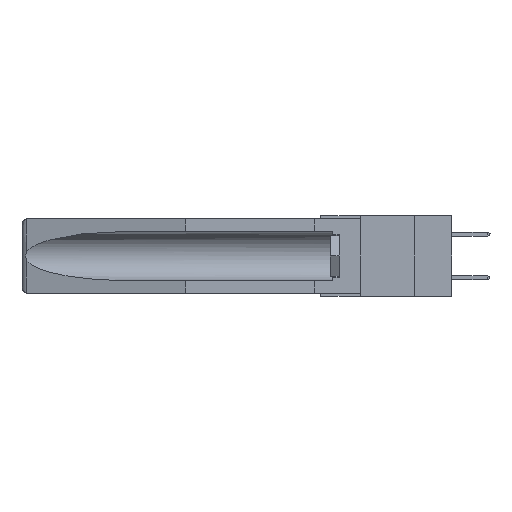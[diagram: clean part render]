
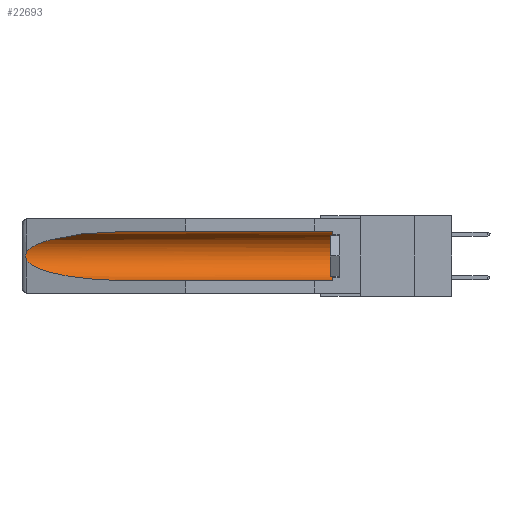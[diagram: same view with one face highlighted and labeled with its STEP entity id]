
A CAD part, left-side view. The second image highlights one B-rep face of the part: STEP entity #22693.
In plain terms, the highlighted cylindrical face has radius 2.857 mm (diameter 5.715 mm), a partial arc.
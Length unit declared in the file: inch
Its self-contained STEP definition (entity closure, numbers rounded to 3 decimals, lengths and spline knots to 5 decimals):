
#104 = DIRECTION ( 'NONE',  ( 0., 0., 1. ) ) ;
#618 = VERTEX_POINT ( 'NONE', #13169 ) ;
#2850 = AXIS2_PLACEMENT_3D ( 'NONE', #29302, #12072, #104 ) ;
#3590 = VERTEX_POINT ( 'NONE', #14461 ) ;
#4491 = EDGE_CURVE ( 'NONE', #618, #12847, #23734, .T. ) ;
#5005 = DIRECTION ( 'NONE',  ( 0., 1., 0. ) ) ;
#6200 = ORIENTED_EDGE ( 'NONE', *, *, #6439, .T. ) ;
#6439 = EDGE_CURVE ( 'NONE', #16627, #12847, #22636, .T. ) ;
#6480 = CARTESIAN_POINT ( 'NONE',  ( 0.21114, 1.30732, -0.059 ) ) ;
#6507 = CARTESIAN_POINT ( 'NONE',  ( 0.26537, 1.52718, -0.19328 ) ) ;
#8005 = LINE ( 'NONE', #29593, #15576 ) ;
#9038 = CARTESIAN_POINT ( 'NONE',  ( 0.155, -0.30754, -0.284 ) ) ;
#10639 = CARTESIAN_POINT ( 'NONE',  ( 0.155, 1.07973, -0.284 ) ) ;
#10770 = EDGE_LOOP ( 'NONE', ( #22137, #22487, #6200, #28741, #30874, #13702 ) ) ;
#10955 = CARTESIAN_POINT ( 'NONE',  ( 0.2673, 1.53269, -0.17917 ) ) ;
#11269 = CARTESIAN_POINT ( 'NONE',  ( 0.26655, 1.53094, -0.18657 ) ) ;
#11281 = VECTOR ( 'NONE', #30518, 39.37008 ) ;
#12072 = DIRECTION ( 'NONE',  ( 0., -1., 0. ) ) ;
#12361 = EDGE_CURVE ( 'NONE', #618, #3590, #28102, .T. ) ;
#12847 = VERTEX_POINT ( 'NONE', #10639 ) ;
#12888 = DIRECTION ( 'NONE',  ( 0., 1., 0. ) ) ;
#13169 = CARTESIAN_POINT ( 'NONE',  ( 0.155, 0.126, -0.284 ) ) ;
#13183 = CARTESIAN_POINT ( 'NONE',  ( 0.26597, 1.52961, -0.15275 ) ) ;
#13702 = ORIENTED_EDGE ( 'NONE', *, *, #24651, .T. ) ;
#14461 = CARTESIAN_POINT ( 'NONE',  ( 0.155, 0.126, -0.059 ) ) ;
#15488 = CARTESIAN_POINT ( 'NONE',  ( 0.26537, 1.52718, -0.19328 ) ) ;
#15576 = VECTOR ( 'NONE', #12888, 39.37008 ) ;
#15831 = CARTESIAN_POINT ( 'NONE',  ( 0.26537, 1.52718, -0.19328 ) ) ;
#16154 = CARTESIAN_POINT ( 'NONE',  ( 0.26597, 1.5296, -0.19026 ) ) ;
#16467 =( BOUNDED_CURVE ( )  B_SPLINE_CURVE ( 3, ( #31258, #6480, #23387, #16859 ),
 .UNSPECIFIED., .F., .T. ) 
 B_SPLINE_CURVE_WITH_KNOTS ( ( 4, 4 ),
 ( 4.71239, 6.08839 ),
 .UNSPECIFIED. ) 
 CURVE ( )  GEOMETRIC_REPRESENTATION_ITEM ( )  RATIONAL_B_SPLINE_CURVE ( ( 1., 0.848, 0.848, 1. ) ) 
 REPRESENTATION_ITEM ( '' )  );
#16627 = VERTEX_POINT ( 'NONE', #15488 ) ;
#16859 = CARTESIAN_POINT ( 'NONE',  ( 0.26537, 1.52718, -0.14972 ) ) ;
#17693 = EDGE_CURVE ( 'NONE', #24931, #26685, #16467, .T. ) ;
#17947 = CARTESIAN_POINT ( 'NONE',  ( 0.26537, 1.52718, -0.14972 ) ) ;
#19496 = EDGE_CURVE ( 'NONE', #26685, #16627, #21074, .T. ) ;
#19726 = CARTESIAN_POINT ( 'NONE',  ( 0.155, -0.30754, -0.1715 ) ) ;
#20788 = CARTESIAN_POINT ( 'NONE',  ( 0.2675, 1.53308, -0.16763 ) ) ;
#20820 = CARTESIAN_POINT ( 'NONE',  ( 0.26537, 1.52718, -0.14972 ) ) ;
#21074 = B_SPLINE_CURVE_WITH_KNOTS ( 'NONE', 3,
 ( #17947, #13183, #28186, #30318, #20788, #25516, #10955, #11269, #16154, #6507 ),
 .UNSPECIFIED., .F., .F.,
 ( 4, 2, 2, 2, 4 ),
 ( 0., 0.00029, 0.00058, 0.00087, 0.00117 ),
 .UNSPECIFIED. ) ;
#22137 = ORIENTED_EDGE ( 'NONE', *, *, #17693, .T. ) ;
#22348 = DIRECTION ( 'NONE',  ( 0., 0., 1. ) ) ;
#22487 = ORIENTED_EDGE ( 'NONE', *, *, #19496, .T. ) ;
#22636 =( BOUNDED_CURVE ( )  B_SPLINE_CURVE ( 3, ( #15831, #27751, #25714, #27970 ),
 .UNSPECIFIED., .F., .F. ) 
 B_SPLINE_CURVE_WITH_KNOTS ( ( 4, 4 ),
 ( 0.1948, 1.5708 ),
 .UNSPECIFIED. ) 
 CURVE ( )  GEOMETRIC_REPRESENTATION_ITEM ( )  RATIONAL_B_SPLINE_CURVE ( ( 1., 0.848, 0.848, 1. ) ) 
 REPRESENTATION_ITEM ( '' )  );
#22693 = ADVANCED_FACE ( 'NONE', ( #28158 ), #24349, .F. ) ;
#23387 = CARTESIAN_POINT ( 'NONE',  ( 0.25451, 1.48313, -0.09465 ) ) ;
#23734 = LINE ( 'NONE', #9038, #11281 ) ;
#24349 = CYLINDRICAL_SURFACE ( 'NONE', #30832, 0.1125 ) ;
#24651 = EDGE_CURVE ( 'NONE', #3590, #24931, #8005, .T. ) ;
#24931 = VERTEX_POINT ( 'NONE', #31096 ) ;
#25516 = CARTESIAN_POINT ( 'NONE',  ( 0.2675, 1.53308, -0.17534 ) ) ;
#25714 = CARTESIAN_POINT ( 'NONE',  ( 0.21114, 1.30732, -0.284 ) ) ;
#26685 = VERTEX_POINT ( 'NONE', #20820 ) ;
#27751 = CARTESIAN_POINT ( 'NONE',  ( 0.25451, 1.48313, -0.24835 ) ) ;
#27970 = CARTESIAN_POINT ( 'NONE',  ( 0.155, 1.07973, -0.284 ) ) ;
#28102 = CIRCLE ( 'NONE', #2850, 0.1125 ) ;
#28158 = FACE_OUTER_BOUND ( 'NONE', #10770, .T. ) ;
#28186 = CARTESIAN_POINT ( 'NONE',  ( 0.26654, 1.53092, -0.15636 ) ) ;
#28741 = ORIENTED_EDGE ( 'NONE', *, *, #4491, .F. ) ;
#29302 = CARTESIAN_POINT ( 'NONE',  ( 0.155, 0.126, -0.1715 ) ) ;
#29593 = CARTESIAN_POINT ( 'NONE',  ( 0.155, -0.30754, -0.059 ) ) ;
#30318 = CARTESIAN_POINT ( 'NONE',  ( 0.2673, 1.5327, -0.16383 ) ) ;
#30518 = DIRECTION ( 'NONE',  ( 0., 1., 0. ) ) ;
#30832 = AXIS2_PLACEMENT_3D ( 'NONE', #19726, #5005, #22348 ) ;
#30874 = ORIENTED_EDGE ( 'NONE', *, *, #12361, .T. ) ;
#31096 = CARTESIAN_POINT ( 'NONE',  ( 0.155, 1.07973, -0.059 ) ) ;
#31258 = CARTESIAN_POINT ( 'NONE',  ( 0.155, 1.07973, -0.059 ) ) ;
